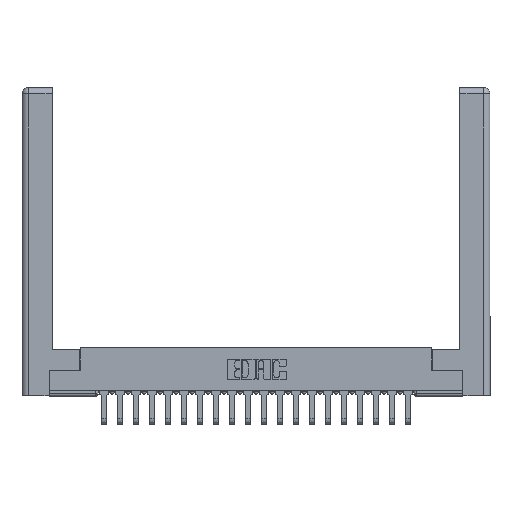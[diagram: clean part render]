
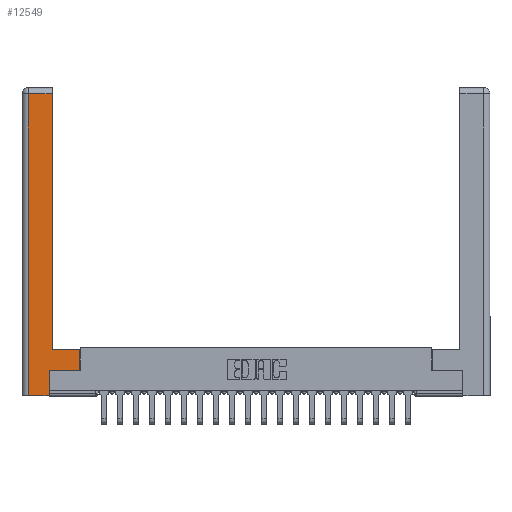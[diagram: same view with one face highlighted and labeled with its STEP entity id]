
A CAD part, top view. The second image highlights one B-rep face of the part: STEP entity #12549.
In plain terms, the highlighted planar face has unit normal (0, 0, 1).
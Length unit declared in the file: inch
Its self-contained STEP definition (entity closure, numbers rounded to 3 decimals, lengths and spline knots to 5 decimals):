
#284 = CARTESIAN_POINT ( 'NONE',  ( 0.295, 2.94, 0. ) ) ;
#727 = DIRECTION ( 'NONE',  ( 0., 0., -1. ) ) ;
#892 = ORIENTED_EDGE ( 'NONE', *, *, #7449, .T. ) ;
#1034 = VERTEX_POINT ( 'NONE', #2563 ) ;
#1908 = CARTESIAN_POINT ( 'NONE',  ( 0.265, 0., 0. ) ) ;
#2259 = LINE ( 'NONE', #15708, #18707 ) ;
#2563 = CARTESIAN_POINT ( 'NONE',  ( 0.0615, 0., 0. ) ) ;
#3430 = VERTEX_POINT ( 'NONE', #4904 ) ;
#3500 = ORIENTED_EDGE ( 'NONE', *, *, #5625, .T. ) ;
#4267 = CARTESIAN_POINT ( 'NONE',  ( 0.565, 0.45, 0. ) ) ;
#4478 = LINE ( 'NONE', #8707, #8828 ) ;
#4500 = CARTESIAN_POINT ( 'NONE',  ( 0.295, 0.45, 0. ) ) ;
#4904 = CARTESIAN_POINT ( 'NONE',  ( 0.565, 0.245, 0. ) ) ;
#5127 = LINE ( 'NONE', #17961, #13839 ) ;
#5243 = VECTOR ( 'NONE', #13143, 39.37008 ) ;
#5625 = EDGE_CURVE ( 'NONE', #22263, #9156, #4478, .T. ) ;
#5789 = CARTESIAN_POINT ( 'NONE',  ( 0.565, 0.45, 0. ) ) ;
#6046 = EDGE_CURVE ( 'NONE', #14965, #22263, #19901, .T. ) ;
#7449 = EDGE_CURVE ( 'NONE', #3430, #14965, #13751, .T. ) ;
#7794 = VERTEX_POINT ( 'NONE', #19443 ) ;
#8314 = CARTESIAN_POINT ( 'NONE',  ( 0.0615, 2.94, 0. ) ) ;
#8707 = CARTESIAN_POINT ( 'NONE',  ( 0.295, 3., 0. ) ) ;
#8828 = VECTOR ( 'NONE', #12089, 39.37008 ) ;
#9156 = VERTEX_POINT ( 'NONE', #284 ) ;
#9692 = CARTESIAN_POINT ( 'NONE',  ( 0.265, 0.245, 0. ) ) ;
#10413 = DIRECTION ( 'NONE',  ( -1., 0., 0. ) ) ;
#10682 = LINE ( 'NONE', #18270, #16700 ) ;
#11021 = LINE ( 'NONE', #1908, #5243 ) ;
#11877 = DIRECTION ( 'NONE',  ( 0., 1., 0. ) ) ;
#12089 = DIRECTION ( 'NONE',  ( 0., 1., 0. ) ) ;
#12302 = CARTESIAN_POINT ( 'NONE',  ( 0.295, 0.45, 0. ) ) ;
#12433 = LINE ( 'NONE', #20039, #24301 ) ;
#12549 = ADVANCED_FACE ( 'NONE', ( #21782 ), #17793, .F. ) ;
#13143 = DIRECTION ( 'NONE',  ( 1., 0., 0. ) ) ;
#13751 = LINE ( 'NONE', #4267, #15318 ) ;
#13839 = VECTOR ( 'NONE', #23696, 39.37008 ) ;
#14965 = VERTEX_POINT ( 'NONE', #5789 ) ;
#15318 = VECTOR ( 'NONE', #11877, 39.37008 ) ;
#15704 = EDGE_CURVE ( 'NONE', #16361, #3430, #5127, .T. ) ;
#15708 = CARTESIAN_POINT ( 'NONE',  ( 0.0615, 2.94, 0. ) ) ;
#15919 = DIRECTION ( 'NONE',  ( -1., 0., 0. ) ) ;
#16361 = VERTEX_POINT ( 'NONE', #9692 ) ;
#16700 = VECTOR ( 'NONE', #24006, 39.37008 ) ;
#16751 = VECTOR ( 'NONE', #10413, 39.37008 ) ;
#16876 = EDGE_LOOP ( 'NONE', ( #3500, #21523, #21614, #21179, #23516, #19957, #892, #20319 ) ) ;
#17793 = PLANE ( 'NONE',  #21310 ) ;
#17929 = EDGE_CURVE ( 'NONE', #7794, #16361, #10682, .T. ) ;
#17961 = CARTESIAN_POINT ( 'NONE',  ( 0.565, 0.245, 0. ) ) ;
#18146 = DIRECTION ( 'NONE',  ( 0., -1., 0. ) ) ;
#18270 = CARTESIAN_POINT ( 'NONE',  ( 0.265, 0.245, 0. ) ) ;
#18519 = EDGE_CURVE ( 'NONE', #9156, #20678, #2259, .T. ) ;
#18707 = VECTOR ( 'NONE', #23428, 39.37008 ) ;
#19443 = CARTESIAN_POINT ( 'NONE',  ( 0.265, 0., 0. ) ) ;
#19568 = EDGE_CURVE ( 'NONE', #20678, #1034, #12433, .T. ) ;
#19901 = LINE ( 'NONE', #12302, #16751 ) ;
#19957 = ORIENTED_EDGE ( 'NONE', *, *, #15704, .T. ) ;
#20039 = CARTESIAN_POINT ( 'NONE',  ( 0.0615, 0., 0. ) ) ;
#20048 = CARTESIAN_POINT ( 'NONE',  ( 0., 0., 0. ) ) ;
#20195 = EDGE_CURVE ( 'NONE', #1034, #7794, #11021, .T. ) ;
#20319 = ORIENTED_EDGE ( 'NONE', *, *, #6046, .T. ) ;
#20678 = VERTEX_POINT ( 'NONE', #8314 ) ;
#21179 = ORIENTED_EDGE ( 'NONE', *, *, #20195, .T. ) ;
#21310 = AXIS2_PLACEMENT_3D ( 'NONE', #20048, #727, #15919 ) ;
#21523 = ORIENTED_EDGE ( 'NONE', *, *, #18519, .T. ) ;
#21614 = ORIENTED_EDGE ( 'NONE', *, *, #19568, .T. ) ;
#21782 = FACE_OUTER_BOUND ( 'NONE', #16876, .T. ) ;
#22263 = VERTEX_POINT ( 'NONE', #4500 ) ;
#23428 = DIRECTION ( 'NONE',  ( -1., 0., 0. ) ) ;
#23516 = ORIENTED_EDGE ( 'NONE', *, *, #17929, .T. ) ;
#23696 = DIRECTION ( 'NONE',  ( 1., 0., 0. ) ) ;
#24006 = DIRECTION ( 'NONE',  ( 0., 1., 0. ) ) ;
#24301 = VECTOR ( 'NONE', #18146, 39.37008 ) ;
